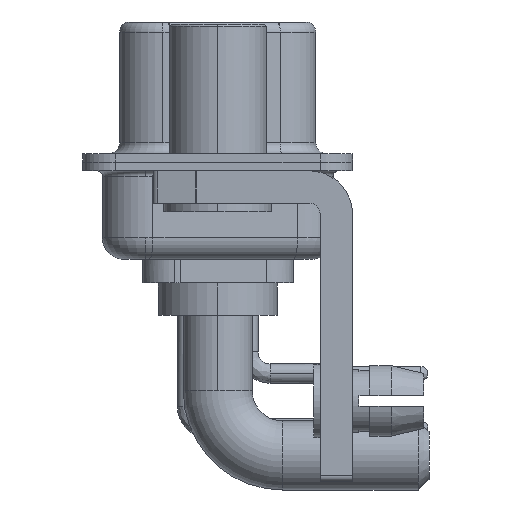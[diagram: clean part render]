
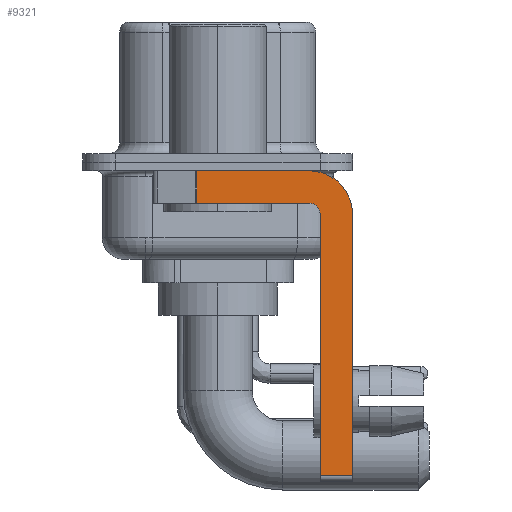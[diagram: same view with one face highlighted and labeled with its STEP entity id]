
A CAD part, left-side view. The second image highlights one B-rep face of the part: STEP entity #9321.
In plain terms, the highlighted planar face has unit normal (-1, 0, 0).
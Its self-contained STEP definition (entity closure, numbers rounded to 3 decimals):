
#43 = CARTESIAN_POINT ( 'NONE',  ( -2.9, -6.25, -14.55 ) ) ;
#622 = ORIENTED_EDGE ( 'NONE', *, *, #21542, .F. ) ;
#684 = AXIS2_PLACEMENT_3D ( 'NONE', #12497, #5825, #26097 ) ;
#895 = LINE ( 'NONE', #7545, #13189 ) ;
#1607 = ORIENTED_EDGE ( 'NONE', *, *, #9609, .F. ) ;
#1862 = CARTESIAN_POINT ( 'NONE',  ( -2.9, -4.25, -14.55 ) ) ;
#3795 = ORIENTED_EDGE ( 'NONE', *, *, #20644, .F. ) ;
#4537 = LINE ( 'NONE', #22195, #28487 ) ;
#4715 = ORIENTED_EDGE ( 'NONE', *, *, #21821, .T. ) ;
#4739 = VECTOR ( 'NONE', #26790, 1000. ) ;
#5039 = ORIENTED_EDGE ( 'NONE', *, *, #12439, .F. ) ;
#5150 = EDGE_CURVE ( 'NONE', #26445, #12560, #4537, .T. ) ;
#5505 = CARTESIAN_POINT ( 'NONE',  ( -2.9, -4.25, -2.4 ) ) ;
#5550 = CARTESIAN_POINT ( 'NONE',  ( -2.9, -4.75, -14.8 ) ) ;
#5825 = DIRECTION ( 'NONE',  ( 1., 0., 0. ) ) ;
#5878 = ORIENTED_EDGE ( 'NONE', *, *, #28081, .F. ) ;
#6468 = VERTEX_POINT ( 'NONE', #26978 ) ;
#6735 = CIRCLE ( 'NONE', #19660, 2. ) ;
#6861 = DIRECTION ( 'NONE',  ( 0., 0., -1. ) ) ;
#7545 = CARTESIAN_POINT ( 'NONE',  ( -2.9, -4.25, -1.9 ) ) ;
#7894 = VERTEX_POINT ( 'NONE', #18977 ) ;
#8071 = VERTEX_POINT ( 'NONE', #9265 ) ;
#8591 = PLANE ( 'NONE',  #684 ) ;
#9265 = CARTESIAN_POINT ( 'NONE',  ( -2.9, -4.25, -0.4 ) ) ;
#9321 = ADVANCED_FACE ( 'NONE', ( #18981 ), #8591, .F. ) ;
#9588 = DIRECTION ( 'NONE',  ( -1., 0., 0. ) ) ;
#9609 = EDGE_CURVE ( 'NONE', #6468, #24563, #13608, .T. ) ;
#9781 = DIRECTION ( 'NONE',  ( 0., 0., 1. ) ) ;
#9799 = DIRECTION ( 'NONE',  ( 0., 0., -1. ) ) ;
#11218 = VECTOR ( 'NONE', #9781, 1000. ) ;
#11485 = CARTESIAN_POINT ( 'NONE',  ( -2.9, -6.25, -2.4 ) ) ;
#12220 = AXIS2_PLACEMENT_3D ( 'NONE', #5505, #9588, #23026 ) ;
#12439 = EDGE_CURVE ( 'NONE', #8071, #15923, #6735, .T. ) ;
#12497 = CARTESIAN_POINT ( 'NONE',  ( -2.9, -4.25, -2.4 ) ) ;
#12560 = VERTEX_POINT ( 'NONE', #14412 ) ;
#13174 = CARTESIAN_POINT ( 'NONE',  ( -2.9, 0.978, -0.4 ) ) ;
#13189 = VECTOR ( 'NONE', #16364, 1000. ) ;
#13293 = DIRECTION ( 'NONE',  ( 0., -1., 0. ) ) ;
#13608 = CIRCLE ( 'NONE', #12220, 0.5 ) ;
#13897 = CARTESIAN_POINT ( 'NONE',  ( -2.9, 3., -0.4 ) ) ;
#13953 = ORIENTED_EDGE ( 'NONE', *, *, #5150, .T. ) ;
#14096 = DIRECTION ( 'NONE',  ( 0., 0., -1. ) ) ;
#14116 = LINE ( 'NONE', #5550, #11218 ) ;
#14412 = CARTESIAN_POINT ( 'NONE',  ( -2.9, 0.978, -1.9 ) ) ;
#15923 = VERTEX_POINT ( 'NONE', #11485 ) ;
#16313 = ORIENTED_EDGE ( 'NONE', *, *, #26329, .F. ) ;
#16364 = DIRECTION ( 'NONE',  ( 0., 1., 0. ) ) ;
#16430 = DIRECTION ( 'NONE',  ( 1., 0., 0. ) ) ;
#16526 = CARTESIAN_POINT ( 'NONE',  ( -2.9, -6.25, -2.4 ) ) ;
#17006 = CARTESIAN_POINT ( 'NONE',  ( -2.9, -4.25, -2.4 ) ) ;
#18977 = CARTESIAN_POINT ( 'NONE',  ( -2.9, -4.75, -14.55 ) ) ;
#18981 = FACE_OUTER_BOUND ( 'NONE', #26501, .T. ) ;
#19660 = AXIS2_PLACEMENT_3D ( 'NONE', #17006, #16430, #9799 ) ;
#20644 = EDGE_CURVE ( 'NONE', #7894, #6468, #14116, .T. ) ;
#21542 = EDGE_CURVE ( 'NONE', #26445, #8071, #22714, .T. ) ;
#21821 = EDGE_CURVE ( 'NONE', #7894, #26014, #24449, .T. ) ;
#22033 = CARTESIAN_POINT ( 'NONE',  ( -2.9, -4.25, -1.9 ) ) ;
#22054 = VECTOR ( 'NONE', #14096, 1000. ) ;
#22195 = CARTESIAN_POINT ( 'NONE',  ( -2.9, 0.978, -1.9 ) ) ;
#22714 = LINE ( 'NONE', #13897, #4739 ) ;
#22750 = VECTOR ( 'NONE', #13293, 1000. ) ;
#23026 = DIRECTION ( 'NONE',  ( 0., 0., 1. ) ) ;
#24449 = LINE ( 'NONE', #1862, #22750 ) ;
#24563 = VERTEX_POINT ( 'NONE', #22033 ) ;
#26014 = VERTEX_POINT ( 'NONE', #43 ) ;
#26097 = DIRECTION ( 'NONE',  ( 0., 0., -1. ) ) ;
#26329 = EDGE_CURVE ( 'NONE', #24563, #12560, #895, .T. ) ;
#26445 = VERTEX_POINT ( 'NONE', #13174 ) ;
#26501 = EDGE_LOOP ( 'NONE', ( #622, #13953, #16313, #1607, #3795, #4715, #5878, #5039 ) ) ;
#26790 = DIRECTION ( 'NONE',  ( 0., -1., 0. ) ) ;
#26978 = CARTESIAN_POINT ( 'NONE',  ( -2.9, -4.75, -2.4 ) ) ;
#27549 = LINE ( 'NONE', #16526, #22054 ) ;
#28081 = EDGE_CURVE ( 'NONE', #15923, #26014, #27549, .T. ) ;
#28487 = VECTOR ( 'NONE', #6861, 1000. ) ;
